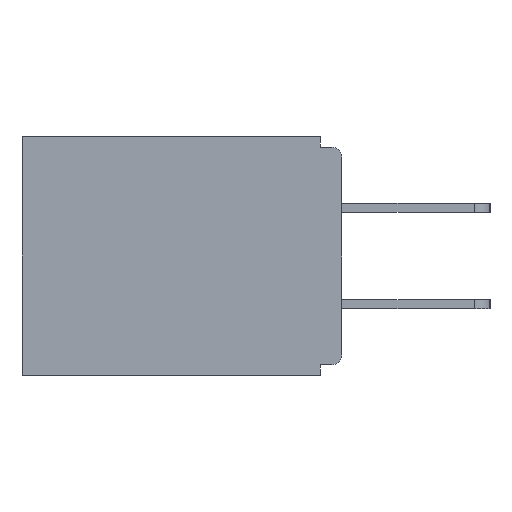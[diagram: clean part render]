
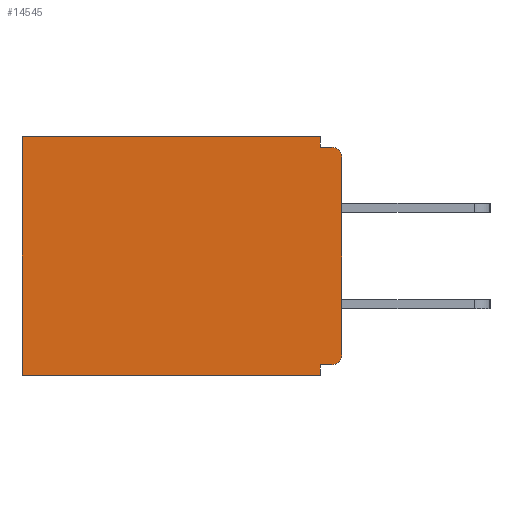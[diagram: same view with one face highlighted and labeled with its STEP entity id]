
A CAD part, left-side view. The second image highlights one B-rep face of the part: STEP entity #14545.
In plain terms, the highlighted planar face has unit normal (-1, 0, 0).
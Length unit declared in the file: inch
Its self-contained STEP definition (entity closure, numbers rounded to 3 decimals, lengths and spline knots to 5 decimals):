
#540 = EDGE_CURVE ( 'NONE', #21250, #11919, #6864, .T. ) ;
#622 = AXIS2_PLACEMENT_3D ( 'NONE', #16874, #2623, #9097 ) ;
#785 = EDGE_CURVE ( 'NONE', #16024, #9343, #4309, .T. ) ;
#1014 = CARTESIAN_POINT ( 'NONE',  ( 0.298, 0.46, 0. ) ) ;
#1148 = CARTESIAN_POINT ( 'NONE',  ( 0.298, 0., 0. ) ) ;
#1241 = EDGE_CURVE ( 'NONE', #12231, #21250, #15157, .T. ) ;
#1514 = DIRECTION ( 'NONE',  ( 1., 0., 0. ) ) ;
#2623 = DIRECTION ( 'NONE',  ( -1., 0., 0. ) ) ;
#2634 = EDGE_CURVE ( 'NONE', #21099, #2656, #2839, .T. ) ;
#2656 = VERTEX_POINT ( 'NONE', #11183 ) ;
#2839 = CIRCLE ( 'NONE', #622, 0.015 ) ;
#2860 = DIRECTION ( 'NONE',  ( 0., 0., -1. ) ) ;
#2937 = AXIS2_PLACEMENT_3D ( 'NONE', #8906, #1514, #8596 ) ;
#2975 = EDGE_CURVE ( 'NONE', #21099, #9343, #4918, .T. ) ;
#3020 = FACE_OUTER_BOUND ( 'NONE', #16276, .T. ) ;
#3708 = VERTEX_POINT ( 'NONE', #8298 ) ;
#3964 = DIRECTION ( 'NONE',  ( 0., 0., -1. ) ) ;
#3980 = DIRECTION ( 'NONE',  ( 0., 1., 0. ) ) ;
#4110 = CARTESIAN_POINT ( 'NONE',  ( 0.298, 0.46, -0.343 ) ) ;
#4309 = CIRCLE ( 'NONE', #17708, 0.015 ) ;
#4757 = LINE ( 'NONE', #8052, #11428 ) ;
#4918 = LINE ( 'NONE', #20117, #21022 ) ;
#4949 = DIRECTION ( 'NONE',  ( 0., 1., 0. ) ) ;
#5011 = ORIENTED_EDGE ( 'NONE', *, *, #20824, .F. ) ;
#5119 = LINE ( 'NONE', #14418, #16794 ) ;
#5162 = ORIENTED_EDGE ( 'NONE', *, *, #6064, .F. ) ;
#6064 = EDGE_CURVE ( 'NONE', #16024, #9131, #4757, .T. ) ;
#6597 = CARTESIAN_POINT ( 'NONE',  ( 0.298, 0.46, 0. ) ) ;
#6864 = LINE ( 'NONE', #1014, #11880 ) ;
#7333 = CARTESIAN_POINT ( 'NONE',  ( 0.298, 0.031, -0.343 ) ) ;
#7404 = CARTESIAN_POINT ( 'NONE',  ( 0.298, 0., -0.03 ) ) ;
#8052 = CARTESIAN_POINT ( 'NONE',  ( 0.298, 0., -0.328 ) ) ;
#8117 = LINE ( 'NONE', #14384, #10898 ) ;
#8298 = CARTESIAN_POINT ( 'NONE',  ( 0.298, 0.031, -0.015 ) ) ;
#8596 = DIRECTION ( 'NONE',  ( 0., 0., -1. ) ) ;
#8901 = VECTOR ( 'NONE', #18102, 39.37008 ) ;
#8906 = CARTESIAN_POINT ( 'NONE',  ( 0.298, 0., 0. ) ) ;
#9097 = DIRECTION ( 'NONE',  ( 0., 0., -1. ) ) ;
#9131 = VERTEX_POINT ( 'NONE', #22035 ) ;
#9343 = VERTEX_POINT ( 'NONE', #18853 ) ;
#9596 = VECTOR ( 'NONE', #4949, 39.37008 ) ;
#10697 = ORIENTED_EDGE ( 'NONE', *, *, #2634, .T. ) ;
#10898 = VECTOR ( 'NONE', #19421, 39.37008 ) ;
#11183 = CARTESIAN_POINT ( 'NONE',  ( 0.298, 0.015, -0.015 ) ) ;
#11428 = VECTOR ( 'NONE', #20377, 39.37008 ) ;
#11880 = VECTOR ( 'NONE', #2860, 39.37008 ) ;
#11919 = VERTEX_POINT ( 'NONE', #4110 ) ;
#12231 = VERTEX_POINT ( 'NONE', #21121 ) ;
#12405 = PLANE ( 'NONE',  #2937 ) ;
#12454 = CARTESIAN_POINT ( 'NONE',  ( 0.298, 0.015, -0.313 ) ) ;
#12616 = VECTOR ( 'NONE', #3980, 39.37008 ) ;
#12683 = DIRECTION ( 'NONE',  ( -1., 0., 0. ) ) ;
#12873 = DIRECTION ( 'NONE',  ( 0., -1., 0. ) ) ;
#13366 = ORIENTED_EDGE ( 'NONE', *, *, #1241, .T. ) ;
#14170 = ORIENTED_EDGE ( 'NONE', *, *, #785, .T. ) ;
#14384 = CARTESIAN_POINT ( 'NONE',  ( 0.298, 0.031, -0.343 ) ) ;
#14405 = CARTESIAN_POINT ( 'NONE',  ( 0.298, 0.031, -0.343 ) ) ;
#14418 = CARTESIAN_POINT ( 'NONE',  ( 0.298, 0., -0.015 ) ) ;
#14545 = ADVANCED_FACE ( 'NONE', ( #3020 ), #12405, .F. ) ;
#15086 = ORIENTED_EDGE ( 'NONE', *, *, #20373, .F. ) ;
#15157 = LINE ( 'NONE', #1148, #9596 ) ;
#15933 = EDGE_CURVE ( 'NONE', #12231, #3708, #18594, .T. ) ;
#16024 = VERTEX_POINT ( 'NONE', #16622 ) ;
#16075 = DIRECTION ( 'NONE',  ( 0., 0., -1. ) ) ;
#16276 = EDGE_LOOP ( 'NONE', ( #10697, #20304, #21553, #13366, #20909, #15086, #5011, #5162, #14170, #22719 ) ) ;
#16622 = CARTESIAN_POINT ( 'NONE',  ( 0.298, 0.015, -0.328 ) ) ;
#16794 = VECTOR ( 'NONE', #12873, 39.37008 ) ;
#16874 = CARTESIAN_POINT ( 'NONE',  ( 0.298, 0.015, -0.03 ) ) ;
#17708 = AXIS2_PLACEMENT_3D ( 'NONE', #12454, #12683, #16075 ) ;
#18102 = DIRECTION ( 'NONE',  ( 0., 0., -1. ) ) ;
#18594 = LINE ( 'NONE', #7333, #8901 ) ;
#18853 = CARTESIAN_POINT ( 'NONE',  ( 0.298, 0., -0.313 ) ) ;
#19421 = DIRECTION ( 'NONE',  ( 0., 0., -1. ) ) ;
#19590 = EDGE_CURVE ( 'NONE', #3708, #2656, #5119, .T. ) ;
#20076 = LINE ( 'NONE', #21672, #12616 ) ;
#20117 = CARTESIAN_POINT ( 'NONE',  ( 0.298, 0., 0. ) ) ;
#20304 = ORIENTED_EDGE ( 'NONE', *, *, #19590, .F. ) ;
#20373 = EDGE_CURVE ( 'NONE', #22278, #11919, #20076, .T. ) ;
#20377 = DIRECTION ( 'NONE',  ( 0., 1., 0. ) ) ;
#20824 = EDGE_CURVE ( 'NONE', #9131, #22278, #8117, .T. ) ;
#20909 = ORIENTED_EDGE ( 'NONE', *, *, #540, .T. ) ;
#21022 = VECTOR ( 'NONE', #3964, 39.37008 ) ;
#21099 = VERTEX_POINT ( 'NONE', #7404 ) ;
#21121 = CARTESIAN_POINT ( 'NONE',  ( 0.298, 0.031, 0. ) ) ;
#21250 = VERTEX_POINT ( 'NONE', #6597 ) ;
#21553 = ORIENTED_EDGE ( 'NONE', *, *, #15933, .F. ) ;
#21672 = CARTESIAN_POINT ( 'NONE',  ( 0.298, 0., -0.343 ) ) ;
#22035 = CARTESIAN_POINT ( 'NONE',  ( 0.298, 0.031, -0.328 ) ) ;
#22278 = VERTEX_POINT ( 'NONE', #14405 ) ;
#22719 = ORIENTED_EDGE ( 'NONE', *, *, #2975, .F. ) ;
